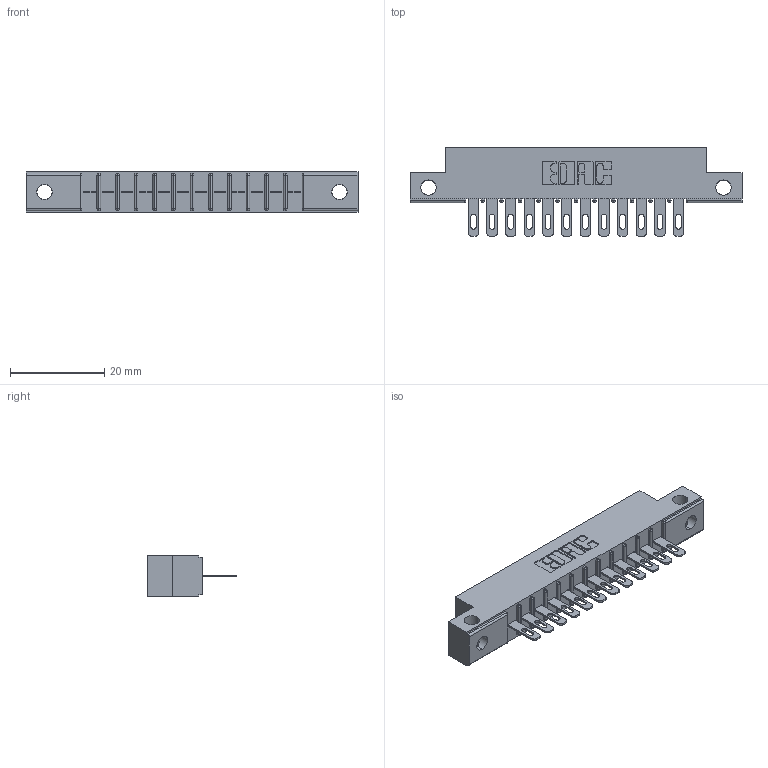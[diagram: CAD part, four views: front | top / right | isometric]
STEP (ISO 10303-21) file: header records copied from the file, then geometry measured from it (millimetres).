
FILE_DESCRIPTION (( 'STEP AP203' ), '1' );
FILE_NAME ('316-012-500-112.STEP', '2020-09-20T20:31:26', ( '' ), ( '' ), 'SwSTEP 2.0', 'SolidWorks 2020', '' );
FILE_SCHEMA (( 'CONFIG_CONTROL_DESIGN' ));
Length unit declared in the file: inch
Products named in the file (3): 306-290-001_100; 306 Part_.128 Dia; 316-012-500-112
Assembly tree (13 placements, depth 2):
  316-012-500-112
    306 Part_.128 Dia
    306-290-001_100  x12
Bounding box: 70.56 x 18.87 x 8.71 mm (x, y, z)
Volume: 4688.8 mm3; surface area: 6743.9 mm2
Topology: 13 solids, 13 shells, 1040 faces, 2932 edges, 1884 vertices
Faces by surface type: plane 668, cylinder 324, sphere 48
Entity records: 15647 total; most frequent: CARTESIAN_POINT 2671, ORIENTED_EDGE 2600, DIRECTION 2576, EDGE_CURVE 1300, LINE 982, VECTOR 982, VERTEX_POINT 828, AXIS2_PLACEMENT_3D 797
